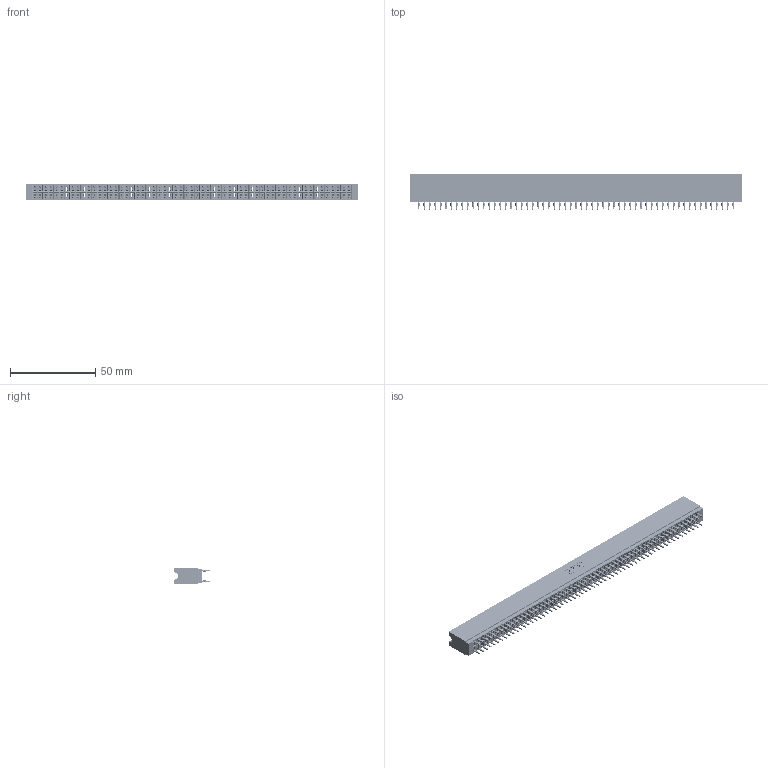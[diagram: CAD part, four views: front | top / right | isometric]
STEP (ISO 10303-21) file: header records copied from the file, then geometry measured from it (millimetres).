
FILE_DESCRIPTION (( 'STEP AP203' ), '1' );
FILE_NAME ('746-118-560-206.STEP', '2026-03-06T17:24:26', ( '' ), ( '' ), 'SwSTEP 2.0', 'SolidWorks 2023', '' );
FILE_SCHEMA (( 'CONFIG_CONTROL_DESIGN' ));
Length unit declared in the file: millimetre
Products named in the file (3): 746-292-001_560; 746-118-560-206; 746 Part_.515 Slot Depth - 06
Assembly tree (119 placements, depth 2):
  746-118-560-206
    746 Part_.515 Slot Depth - 06
    746-292-001_560  x118
Bounding box: 194.56 x 20.82 x 9.91 mm (x, y, z)
Volume: 21131.6 mm3; surface area: 36215.2 mm2
Topology: 119 solids, 119 shells, 11249 faces, 31299 edges, 20058 vertices
Faces by surface type: plane 5602, cylinder 2579, bspline 2360, torus 708
Entity records: 88854 total; most frequent: CARTESIAN_POINT 17512, ORIENTED_EDGE 15330, DIRECTION 12777, EDGE_CURVE 7665, VECTOR 6883, LINE 6883, VERTEX_POINT 5082, AXIS2_PLACEMENT_3D 2947
